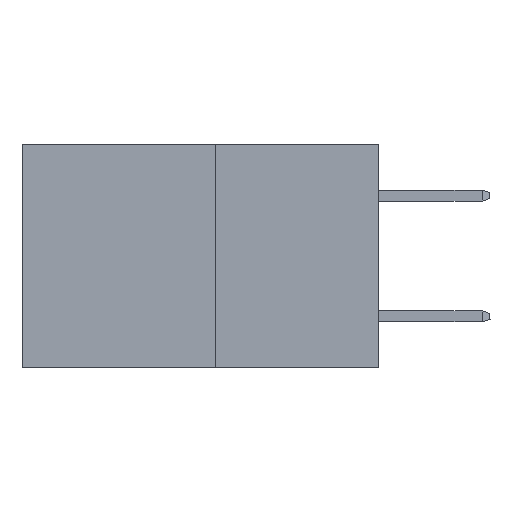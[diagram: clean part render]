
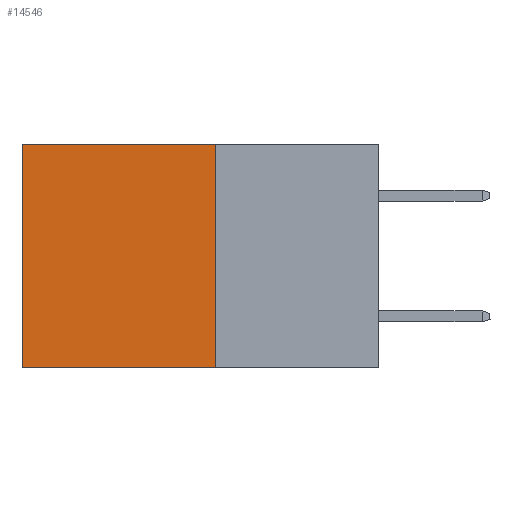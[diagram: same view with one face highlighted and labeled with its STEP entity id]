
A CAD part, left-side view. The second image highlights one B-rep face of the part: STEP entity #14546.
In plain terms, the highlighted planar face has unit normal (-1, 0, 0).
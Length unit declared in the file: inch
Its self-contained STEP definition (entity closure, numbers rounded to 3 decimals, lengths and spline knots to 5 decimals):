
#622 = VECTOR ( 'NONE', #7062, 39.37008 ) ;
#709 = VECTOR ( 'NONE', #1334, 39.37008 ) ;
#836 = EDGE_CURVE ( 'NONE', #19103, #2281, #13645, .T. ) ;
#1334 = DIRECTION ( 'NONE',  ( 0., 0., -1. ) ) ;
#2281 = VERTEX_POINT ( 'NONE', #17529 ) ;
#2385 = DIRECTION ( 'NONE',  ( 0., 0., -1. ) ) ;
#3421 = AXIS2_PLACEMENT_3D ( 'NONE', #12059, #14000, #2385 ) ;
#3960 = CARTESIAN_POINT ( 'NONE',  ( 0.277, 0.59, -0.37 ) ) ;
#4393 = ORIENTED_EDGE ( 'NONE', *, *, #836, .T. ) ;
#4542 = DIRECTION ( 'NONE',  ( 0., 0., -1. ) ) ;
#4757 = VECTOR ( 'NONE', #4542, 39.37008 ) ;
#4967 = DIRECTION ( 'NONE',  ( 0., 1., 0. ) ) ;
#5081 = CARTESIAN_POINT ( 'NONE',  ( 0.277, 0.27, -0.37 ) ) ;
#5781 = LINE ( 'NONE', #5081, #622 ) ;
#6927 = CARTESIAN_POINT ( 'NONE',  ( 0.277, 0.27, 0. ) ) ;
#7062 = DIRECTION ( 'NONE',  ( 0., 1., 0. ) ) ;
#9165 = VERTEX_POINT ( 'NONE', #12470 ) ;
#9989 = ORIENTED_EDGE ( 'NONE', *, *, #22274, .F. ) ;
#10292 = VECTOR ( 'NONE', #4967, 39.37008 ) ;
#11044 = FACE_OUTER_BOUND ( 'NONE', #11247, .T. ) ;
#11247 = EDGE_LOOP ( 'NONE', ( #19441, #9989, #16629, #4393 ) ) ;
#12059 = CARTESIAN_POINT ( 'NONE',  ( 0.277, 0.27, -0.37 ) ) ;
#12470 = CARTESIAN_POINT ( 'NONE',  ( 0.277, 0.27, -0.37 ) ) ;
#13645 = LINE ( 'NONE', #17899, #10292 ) ;
#14000 = DIRECTION ( 'NONE',  ( 1., 0., 0. ) ) ;
#14546 = ADVANCED_FACE ( 'NONE', ( #11044 ), #23547, .F. ) ;
#16159 = LINE ( 'NONE', #24422, #709 ) ;
#16166 = CARTESIAN_POINT ( 'NONE',  ( 0.277, 0.59, -0.37 ) ) ;
#16629 = ORIENTED_EDGE ( 'NONE', *, *, #18734, .F. ) ;
#17529 = CARTESIAN_POINT ( 'NONE',  ( 0.277, 0.59, 0. ) ) ;
#17656 = EDGE_CURVE ( 'NONE', #2281, #22570, #19621, .T. ) ;
#17899 = CARTESIAN_POINT ( 'NONE',  ( 0.277, 0.27, 0. ) ) ;
#18734 = EDGE_CURVE ( 'NONE', #19103, #9165, #16159, .T. ) ;
#19103 = VERTEX_POINT ( 'NONE', #6927 ) ;
#19441 = ORIENTED_EDGE ( 'NONE', *, *, #17656, .T. ) ;
#19621 = LINE ( 'NONE', #16166, #4757 ) ;
#22274 = EDGE_CURVE ( 'NONE', #9165, #22570, #5781, .T. ) ;
#22570 = VERTEX_POINT ( 'NONE', #3960 ) ;
#23547 = PLANE ( 'NONE',  #3421 ) ;
#24422 = CARTESIAN_POINT ( 'NONE',  ( 0.277, 0.27, -0.37 ) ) ;
